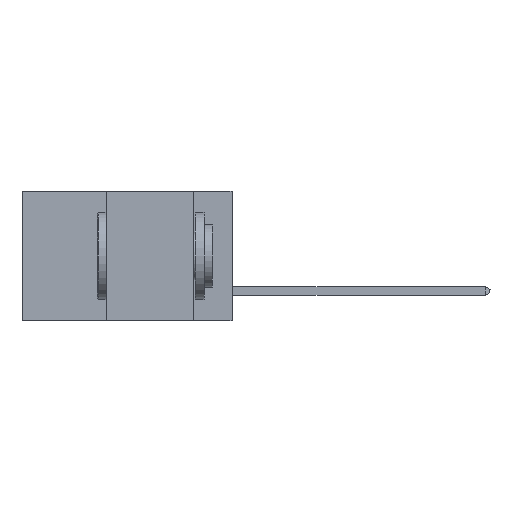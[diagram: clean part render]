
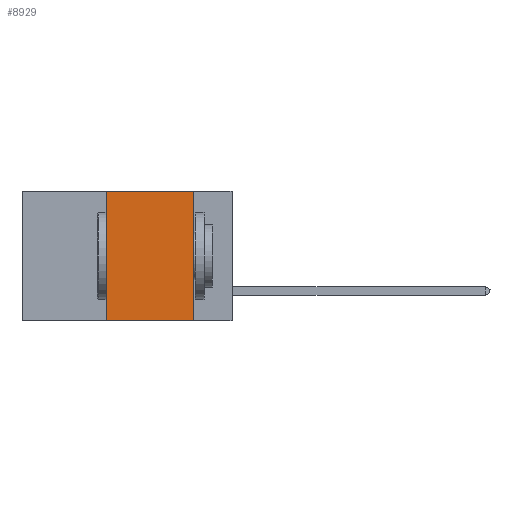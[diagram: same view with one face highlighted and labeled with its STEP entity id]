
A CAD part, left-side view. The second image highlights one B-rep face of the part: STEP entity #8929.
In plain terms, the highlighted planar face has unit normal (-1, 0, 0).
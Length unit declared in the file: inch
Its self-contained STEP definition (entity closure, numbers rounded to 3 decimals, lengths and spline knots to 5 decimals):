
#197 = DIRECTION ( 'NONE',  ( 0., 0., -1. ) ) ;
#718 = ORIENTED_EDGE ( 'NONE', *, *, #12915, .T. ) ;
#982 = VERTEX_POINT ( 'NONE', #9098 ) ;
#995 = CARTESIAN_POINT ( 'NONE',  ( 0., 0.36, 0. ) ) ;
#1285 = LINE ( 'NONE', #8670, #11570 ) ;
#1356 = CARTESIAN_POINT ( 'NONE',  ( 0., 0.36, -0.37 ) ) ;
#2926 = CARTESIAN_POINT ( 'NONE',  ( 0., 0.6, 0. ) ) ;
#2998 = EDGE_CURVE ( 'NONE', #5719, #982, #1285, .T. ) ;
#3038 = DIRECTION ( 'NONE',  ( 1., 0., 0. ) ) ;
#3112 = VERTEX_POINT ( 'NONE', #1356 ) ;
#3292 = LINE ( 'NONE', #8044, #4050 ) ;
#3982 = ORIENTED_EDGE ( 'NONE', *, *, #2998, .F. ) ;
#4050 = VECTOR ( 'NONE', #7896, 39.37008 ) ;
#4285 = LINE ( 'NONE', #10671, #13408 ) ;
#5040 = DIRECTION ( 'NONE',  ( 0., -1., 0. ) ) ;
#5416 = ORIENTED_EDGE ( 'NONE', *, *, #11972, .F. ) ;
#5580 = LINE ( 'NONE', #14969, #10725 ) ;
#5589 = EDGE_LOOP ( 'NONE', ( #3982, #5416, #13004, #718 ) ) ;
#5719 = VERTEX_POINT ( 'NONE', #13044 ) ;
#6331 = EDGE_CURVE ( 'NONE', #3112, #6474, #3292, .T. ) ;
#6474 = VERTEX_POINT ( 'NONE', #995 ) ;
#7437 = AXIS2_PLACEMENT_3D ( 'NONE', #2926, #3038, #15240 ) ;
#7896 = DIRECTION ( 'NONE',  ( 0., 0., 1. ) ) ;
#8044 = CARTESIAN_POINT ( 'NONE',  ( 0., 0.36, 0. ) ) ;
#8670 = CARTESIAN_POINT ( 'NONE',  ( 0., 0.11, 0. ) ) ;
#8929 = ADVANCED_FACE ( 'NONE', ( #10273 ), #13928, .F. ) ;
#9098 = CARTESIAN_POINT ( 'NONE',  ( 0., 0.11, -0.37 ) ) ;
#10273 = FACE_OUTER_BOUND ( 'NONE', #5589, .T. ) ;
#10671 = CARTESIAN_POINT ( 'NONE',  ( 0., 0.6, 0. ) ) ;
#10725 = VECTOR ( 'NONE', #5040, 39.37008 ) ;
#11570 = VECTOR ( 'NONE', #197, 39.37008 ) ;
#11972 = EDGE_CURVE ( 'NONE', #6474, #5719, #4285, .T. ) ;
#12181 = DIRECTION ( 'NONE',  ( 0., -1., 0. ) ) ;
#12915 = EDGE_CURVE ( 'NONE', #3112, #982, #5580, .T. ) ;
#13004 = ORIENTED_EDGE ( 'NONE', *, *, #6331, .F. ) ;
#13044 = CARTESIAN_POINT ( 'NONE',  ( 0., 0.11, 0. ) ) ;
#13408 = VECTOR ( 'NONE', #12181, 39.37008 ) ;
#13928 = PLANE ( 'NONE',  #7437 ) ;
#14969 = CARTESIAN_POINT ( 'NONE',  ( 0., 0.6, -0.37 ) ) ;
#15240 = DIRECTION ( 'NONE',  ( 0., 0., -1. ) ) ;
